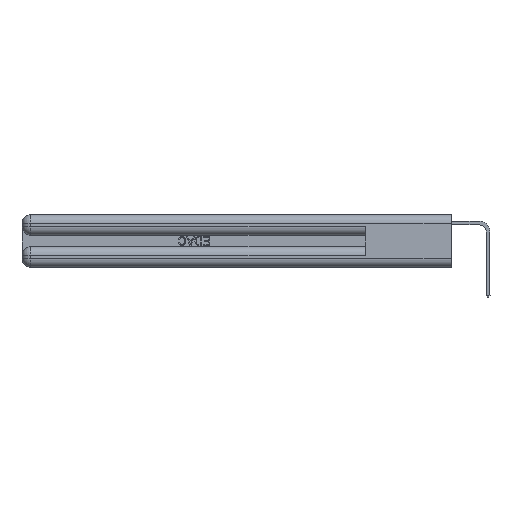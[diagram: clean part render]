
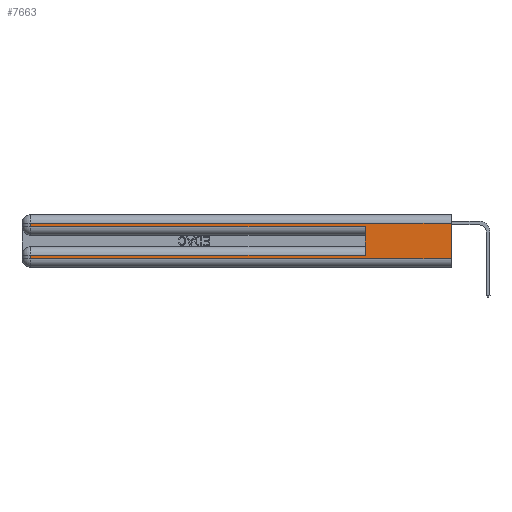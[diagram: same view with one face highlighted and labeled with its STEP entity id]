
A CAD part, left-side view. The second image highlights one B-rep face of the part: STEP entity #7663.
In plain terms, the highlighted planar face has unit normal (-1, 0, 0).
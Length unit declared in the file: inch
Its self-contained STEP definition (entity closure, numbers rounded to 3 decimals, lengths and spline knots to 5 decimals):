
#890 = VERTEX_POINT ( 'NONE', #3448 ) ;
#1676 = VERTEX_POINT ( 'NONE', #4765 ) ;
#2258 = CARTESIAN_POINT ( 'NONE',  ( 0., 2.94, 0.31 ) ) ;
#2360 = LINE ( 'NONE', #18648, #14605 ) ;
#2624 = VERTEX_POINT ( 'NONE', #2258 ) ;
#2660 = DIRECTION ( 'NONE',  ( 0., -1., 0. ) ) ;
#2751 = EDGE_LOOP ( 'NONE', ( #4358, #17936, #27887, #22492, #17284, #28262, #23874, #3210 ) ) ;
#2919 = DIRECTION ( 'NONE',  ( 0., 0., -1. ) ) ;
#3074 = CARTESIAN_POINT ( 'NONE',  ( 0., 0., 0.37 ) ) ;
#3210 = ORIENTED_EDGE ( 'NONE', *, *, #27489, .T. ) ;
#3448 = CARTESIAN_POINT ( 'NONE',  ( 0., 0.6, 0.285 ) ) ;
#3874 = CARTESIAN_POINT ( 'NONE',  ( 0., 0., 0.085 ) ) ;
#4358 = ORIENTED_EDGE ( 'NONE', *, *, #11749, .F. ) ;
#4381 = DIRECTION ( 'NONE',  ( 0., 0., -1. ) ) ;
#4559 = VECTOR ( 'NONE', #2919, 39.37008 ) ;
#4765 = CARTESIAN_POINT ( 'NONE',  ( 0., 0.6, 0.085 ) ) ;
#6307 = DIRECTION ( 'NONE',  ( 0., 1., 0. ) ) ;
#7391 = VECTOR ( 'NONE', #22017, 39.37008 ) ;
#7477 = DIRECTION ( 'NONE',  ( 1., 0., 0. ) ) ;
#7663 = ADVANCED_FACE ( 'NONE', ( #25556 ), #11975, .F. ) ;
#8493 = EDGE_CURVE ( 'NONE', #27763, #890, #21367, .T. ) ;
#10351 = VERTEX_POINT ( 'NONE', #10932 ) ;
#10560 = LINE ( 'NONE', #17304, #7391 ) ;
#10932 = CARTESIAN_POINT ( 'NONE',  ( 0., 0., 0.06 ) ) ;
#11034 = CARTESIAN_POINT ( 'NONE',  ( 0., 2.94, 0.37 ) ) ;
#11481 = LINE ( 'NONE', #11034, #21009 ) ;
#11537 = CARTESIAN_POINT ( 'NONE',  ( 0., 0., 0.37 ) ) ;
#11749 = EDGE_CURVE ( 'NONE', #12447, #10351, #16917, .T. ) ;
#11975 = PLANE ( 'NONE',  #25551 ) ;
#12447 = VERTEX_POINT ( 'NONE', #14121 ) ;
#13662 = EDGE_CURVE ( 'NONE', #2624, #27763, #11481, .T. ) ;
#13677 = CARTESIAN_POINT ( 'NONE',  ( 0., 2.94, 0.085 ) ) ;
#14121 = CARTESIAN_POINT ( 'NONE',  ( 0., 0., 0.31 ) ) ;
#14605 = VECTOR ( 'NONE', #2660, 39.37008 ) ;
#14981 = VECTOR ( 'NONE', #27726, 39.37008 ) ;
#15856 = EDGE_CURVE ( 'NONE', #12447, #2624, #28464, .T. ) ;
#15945 = DIRECTION ( 'NONE',  ( 0., 0., -1. ) ) ;
#16917 = LINE ( 'NONE', #3074, #4559 ) ;
#16977 = CARTESIAN_POINT ( 'NONE',  ( 0., 0., 0.31 ) ) ;
#17284 = ORIENTED_EDGE ( 'NONE', *, *, #22685, .F. ) ;
#17304 = CARTESIAN_POINT ( 'NONE',  ( 0., 0.6, 0.145 ) ) ;
#17936 = ORIENTED_EDGE ( 'NONE', *, *, #15856, .T. ) ;
#18344 = EDGE_CURVE ( 'NONE', #22849, #26730, #29387, .T. ) ;
#18648 = CARTESIAN_POINT ( 'NONE',  ( 0., 0., 0.06 ) ) ;
#21009 = VECTOR ( 'NONE', #4381, 39.37008 ) ;
#21170 = DIRECTION ( 'NONE',  ( 0., 0., -1. ) ) ;
#21367 = LINE ( 'NONE', #25602, #14981 ) ;
#21453 = EDGE_CURVE ( 'NONE', #1676, #22849, #24672, .T. ) ;
#21602 = CARTESIAN_POINT ( 'NONE',  ( 0., 2.94, 0.06 ) ) ;
#22017 = DIRECTION ( 'NONE',  ( 0., 0., 1. ) ) ;
#22492 = ORIENTED_EDGE ( 'NONE', *, *, #8493, .T. ) ;
#22685 = EDGE_CURVE ( 'NONE', #1676, #890, #10560, .T. ) ;
#22849 = VERTEX_POINT ( 'NONE', #13677 ) ;
#23874 = ORIENTED_EDGE ( 'NONE', *, *, #18344, .T. ) ;
#24497 = VECTOR ( 'NONE', #15945, 39.37008 ) ;
#24628 = VECTOR ( 'NONE', #6307, 39.37008 ) ;
#24672 = LINE ( 'NONE', #3874, #24628 ) ;
#25551 = AXIS2_PLACEMENT_3D ( 'NONE', #11537, #7477, #21170 ) ;
#25556 = FACE_OUTER_BOUND ( 'NONE', #2751, .T. ) ;
#25602 = CARTESIAN_POINT ( 'NONE',  ( 0., 0., 0.285 ) ) ;
#26214 = DIRECTION ( 'NONE',  ( 0., 1., 0. ) ) ;
#26730 = VERTEX_POINT ( 'NONE', #21602 ) ;
#26746 = CARTESIAN_POINT ( 'NONE',  ( 0., 2.94, 0.285 ) ) ;
#27149 = CARTESIAN_POINT ( 'NONE',  ( 0., 2.94, 0.37 ) ) ;
#27489 = EDGE_CURVE ( 'NONE', #26730, #10351, #2360, .T. ) ;
#27726 = DIRECTION ( 'NONE',  ( 0., -1., 0. ) ) ;
#27763 = VERTEX_POINT ( 'NONE', #26746 ) ;
#27887 = ORIENTED_EDGE ( 'NONE', *, *, #13662, .T. ) ;
#28262 = ORIENTED_EDGE ( 'NONE', *, *, #21453, .T. ) ;
#28464 = LINE ( 'NONE', #16977, #29215 ) ;
#29215 = VECTOR ( 'NONE', #26214, 39.37008 ) ;
#29387 = LINE ( 'NONE', #27149, #24497 ) ;
